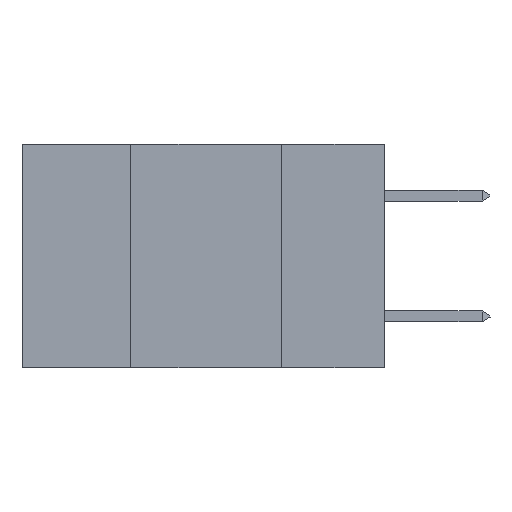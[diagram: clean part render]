
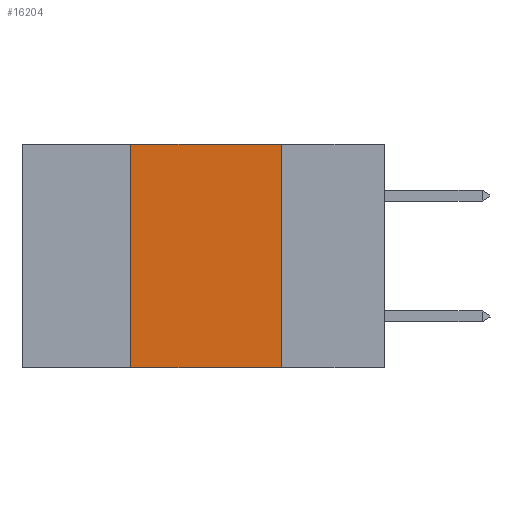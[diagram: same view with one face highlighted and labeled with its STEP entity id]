
A CAD part, left-side view. The second image highlights one B-rep face of the part: STEP entity #16204.
In plain terms, the highlighted planar face has unit normal (-1, 0, 0).
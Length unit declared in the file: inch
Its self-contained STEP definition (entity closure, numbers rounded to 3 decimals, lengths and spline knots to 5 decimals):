
#124 = VERTEX_POINT ( 'NONE', #36167 ) ;
#167 = CARTESIAN_POINT ( 'NONE',  ( 0., 0.6, 0. ) ) ;
#1096 = CARTESIAN_POINT ( 'NONE',  ( 0., 0.17, -0.37 ) ) ;
#2187 = EDGE_CURVE ( 'NONE', #124, #41118, #17492, .T. ) ;
#2317 = DIRECTION ( 'NONE',  ( 0., -1., 0. ) ) ;
#5966 = LINE ( 'NONE', #30356, #11559 ) ;
#6749 = DIRECTION ( 'NONE',  ( 1., 0., 0. ) ) ;
#9537 = ORIENTED_EDGE ( 'NONE', *, *, #2187, .F. ) ;
#10844 = VERTEX_POINT ( 'NONE', #1096 ) ;
#11027 = DIRECTION ( 'NONE',  ( 0., -1., 0. ) ) ;
#11559 = VECTOR ( 'NONE', #17377, 39.37008 ) ;
#16204 = ADVANCED_FACE ( 'NONE', ( #33985 ), #35790, .F. ) ;
#17377 = DIRECTION ( 'NONE',  ( 0., 0., -1. ) ) ;
#17492 = LINE ( 'NONE', #27298, #35868 ) ;
#19404 = EDGE_CURVE ( 'NONE', #124, #10844, #22029, .T. ) ;
#20580 = AXIS2_PLACEMENT_3D ( 'NONE', #167, #6749, #39192 ) ;
#21366 = VERTEX_POINT ( 'NONE', #24577 ) ;
#21885 = EDGE_CURVE ( 'NONE', #21366, #10844, #5966, .T. ) ;
#22029 = LINE ( 'NONE', #24840, #24061 ) ;
#23481 = EDGE_CURVE ( 'NONE', #41118, #21366, #28550, .T. ) ;
#24061 = VECTOR ( 'NONE', #2317, 39.37008 ) ;
#24577 = CARTESIAN_POINT ( 'NONE',  ( 0., 0.17, 0. ) ) ;
#24631 = CARTESIAN_POINT ( 'NONE',  ( 0., 0.6, 0. ) ) ;
#24840 = CARTESIAN_POINT ( 'NONE',  ( 0., 0.6, -0.37 ) ) ;
#27298 = CARTESIAN_POINT ( 'NONE',  ( 0., 0.42, 0. ) ) ;
#27478 = ORIENTED_EDGE ( 'NONE', *, *, #19404, .T. ) ;
#28550 = LINE ( 'NONE', #24631, #38243 ) ;
#30176 = CARTESIAN_POINT ( 'NONE',  ( 0., 0.42, 0. ) ) ;
#30356 = CARTESIAN_POINT ( 'NONE',  ( 0., 0.17, 0. ) ) ;
#32496 = ORIENTED_EDGE ( 'NONE', *, *, #21885, .F. ) ;
#33985 = FACE_OUTER_BOUND ( 'NONE', #34752, .T. ) ;
#34752 = EDGE_LOOP ( 'NONE', ( #32496, #39227, #9537, #27478 ) ) ;
#35790 = PLANE ( 'NONE',  #20580 ) ;
#35868 = VECTOR ( 'NONE', #37412, 39.37008 ) ;
#36167 = CARTESIAN_POINT ( 'NONE',  ( 0., 0.42, -0.37 ) ) ;
#37412 = DIRECTION ( 'NONE',  ( 0., 0., 1. ) ) ;
#38243 = VECTOR ( 'NONE', #11027, 39.37008 ) ;
#39192 = DIRECTION ( 'NONE',  ( 0., 0., -1. ) ) ;
#39227 = ORIENTED_EDGE ( 'NONE', *, *, #23481, .F. ) ;
#41118 = VERTEX_POINT ( 'NONE', #30176 ) ;
